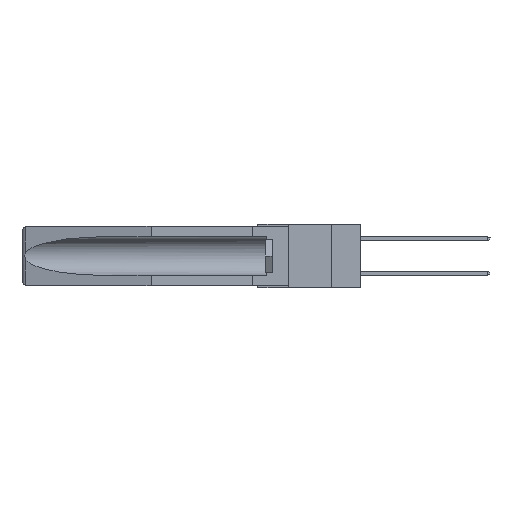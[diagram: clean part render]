
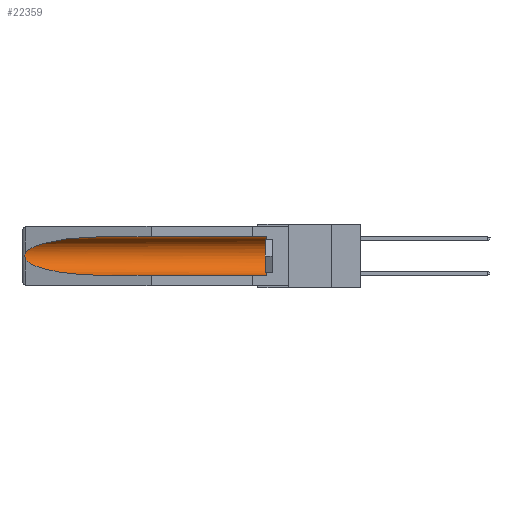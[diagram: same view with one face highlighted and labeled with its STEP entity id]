
A CAD part, left-side view. The second image highlights one B-rep face of the part: STEP entity #22359.
In plain terms, the highlighted cylindrical face has radius 2.857 mm (diameter 5.715 mm), a partial arc.
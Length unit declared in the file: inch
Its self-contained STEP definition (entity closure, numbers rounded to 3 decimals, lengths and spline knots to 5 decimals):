
#38 = ORIENTED_EDGE ( 'NONE', *, *, #10257, .T. ) ;
#1427 = AXIS2_PLACEMENT_3D ( 'NONE', #23069, #27626, #1885 ) ;
#1429 = EDGE_CURVE ( 'NONE', #13107, #6019, #18528, .T. ) ;
#1885 = DIRECTION ( 'NONE',  ( 0., 0., 1. ) ) ;
#2445 = CARTESIAN_POINT ( 'NONE',  ( 0.26537, 1.52718, -0.14972 ) ) ;
#3608 = CARTESIAN_POINT ( 'NONE',  ( 0.26537, 1.52718, -0.14972 ) ) ;
#3795 = CARTESIAN_POINT ( 'NONE',  ( 0.155, -0.30754, -0.284 ) ) ;
#4229 = VERTEX_POINT ( 'NONE', #12191 ) ;
#4608 = CARTESIAN_POINT ( 'NONE',  ( 0.2675, 1.53308, -0.16763 ) ) ;
#4626 = CARTESIAN_POINT ( 'NONE',  ( 0.155, 0.126, -0.284 ) ) ;
#5654 = LINE ( 'NONE', #3795, #27416 ) ;
#6019 = VERTEX_POINT ( 'NONE', #7406 ) ;
#6058 = CARTESIAN_POINT ( 'NONE',  ( 0.155, 1.07973, -0.284 ) ) ;
#6853 = CARTESIAN_POINT ( 'NONE',  ( 0.26597, 1.52961, -0.15275 ) ) ;
#6934 = CARTESIAN_POINT ( 'NONE',  ( 0.2673, 1.5327, -0.16383 ) ) ;
#7406 = CARTESIAN_POINT ( 'NONE',  ( 0.155, 0.126, -0.059 ) ) ;
#7929 = VERTEX_POINT ( 'NONE', #20129 ) ;
#8015 = ORIENTED_EDGE ( 'NONE', *, *, #17765, .T. ) ;
#8219 = DIRECTION ( 'NONE',  ( 0., 1., 0. ) ) ;
#8645 = CARTESIAN_POINT ( 'NONE',  ( 0.21114, 1.30732, -0.059 ) ) ;
#9231 = AXIS2_PLACEMENT_3D ( 'NONE', #27936, #21103, #23392 ) ;
#9607 = VERTEX_POINT ( 'NONE', #3608 ) ;
#10202 = EDGE_CURVE ( 'NONE', #6019, #7929, #25966, .T. ) ;
#10257 = EDGE_CURVE ( 'NONE', #9607, #19282, #23109, .T. ) ;
#10764 =( BOUNDED_CURVE ( )  B_SPLINE_CURVE ( 3, ( #17662, #8645, #13147, #21856 ),
 .UNSPECIFIED., .F., .F. ) 
 B_SPLINE_CURVE_WITH_KNOTS ( ( 4, 4 ),
 ( 4.71239, 6.08839 ),
 .UNSPECIFIED. ) 
 CURVE ( )  GEOMETRIC_REPRESENTATION_ITEM ( )  RATIONAL_B_SPLINE_CURVE ( ( 1., 0.848, 0.848, 1. ) ) 
 REPRESENTATION_ITEM ( '' )  );
#11072 = ORIENTED_EDGE ( 'NONE', *, *, #26405, .T. ) ;
#11145 = DIRECTION ( 'NONE',  ( 0., 1., 0. ) ) ;
#11305 = CARTESIAN_POINT ( 'NONE',  ( 0.2675, 1.53308, -0.17534 ) ) ;
#12184 =( BOUNDED_CURVE ( )  B_SPLINE_CURVE ( 3, ( #19154, #17029, #19353, #6058 ),
 .UNSPECIFIED., .F., .F. ) 
 B_SPLINE_CURVE_WITH_KNOTS ( ( 4, 4 ),
 ( 0.1948, 1.5708 ),
 .UNSPECIFIED. ) 
 CURVE ( )  GEOMETRIC_REPRESENTATION_ITEM ( )  RATIONAL_B_SPLINE_CURVE ( ( 1., 0.848, 0.848, 1. ) ) 
 REPRESENTATION_ITEM ( '' )  );
#12191 = CARTESIAN_POINT ( 'NONE',  ( 0.155, 1.07973, -0.284 ) ) ;
#13107 = VERTEX_POINT ( 'NONE', #4626 ) ;
#13147 = CARTESIAN_POINT ( 'NONE',  ( 0.25451, 1.48313, -0.09465 ) ) ;
#14071 = ORIENTED_EDGE ( 'NONE', *, *, #26380, .F. ) ;
#15782 = CARTESIAN_POINT ( 'NONE',  ( 0.26655, 1.53094, -0.18657 ) ) ;
#17029 = CARTESIAN_POINT ( 'NONE',  ( 0.25451, 1.48313, -0.24835 ) ) ;
#17662 = CARTESIAN_POINT ( 'NONE',  ( 0.155, 1.07973, -0.059 ) ) ;
#17765 = EDGE_CURVE ( 'NONE', #19282, #4229, #12184, .T. ) ;
#17915 = CARTESIAN_POINT ( 'NONE',  ( 0.26654, 1.53092, -0.15636 ) ) ;
#18528 = CIRCLE ( 'NONE', #9231, 0.1125 ) ;
#19154 = CARTESIAN_POINT ( 'NONE',  ( 0.26537, 1.52718, -0.19328 ) ) ;
#19282 = VERTEX_POINT ( 'NONE', #26618 ) ;
#19353 = CARTESIAN_POINT ( 'NONE',  ( 0.21114, 1.30732, -0.284 ) ) ;
#19820 = VECTOR ( 'NONE', #8219, 39.37008 ) ;
#20000 = ORIENTED_EDGE ( 'NONE', *, *, #10202, .T. ) ;
#20115 = CARTESIAN_POINT ( 'NONE',  ( 0.26537, 1.52718, -0.19328 ) ) ;
#20129 = CARTESIAN_POINT ( 'NONE',  ( 0.155, 1.07973, -0.059 ) ) ;
#21103 = DIRECTION ( 'NONE',  ( 0., -1., 0. ) ) ;
#21434 = CARTESIAN_POINT ( 'NONE',  ( 0.155, -0.30754, -0.059 ) ) ;
#21519 = FACE_OUTER_BOUND ( 'NONE', #26461, .T. ) ;
#21856 = CARTESIAN_POINT ( 'NONE',  ( 0.26537, 1.52718, -0.14972 ) ) ;
#22359 = ADVANCED_FACE ( 'NONE', ( #21519 ), #23535, .F. ) ;
#22988 = ORIENTED_EDGE ( 'NONE', *, *, #1429, .T. ) ;
#23069 = CARTESIAN_POINT ( 'NONE',  ( 0.155, -0.30754, -0.1715 ) ) ;
#23109 = B_SPLINE_CURVE_WITH_KNOTS ( 'NONE', 3,
 ( #2445, #6853, #17915, #6934, #4608, #11305, #26731, #15782, #24589, #20115 ),
 .UNSPECIFIED., .F., .F.,
 ( 4, 2, 2, 2, 4 ),
 ( 0., 0.00029, 0.00058, 0.00087, 0.00117 ),
 .UNSPECIFIED. ) ;
#23392 = DIRECTION ( 'NONE',  ( 0., 0., 1. ) ) ;
#23535 = CYLINDRICAL_SURFACE ( 'NONE', #1427, 0.1125 ) ;
#24589 = CARTESIAN_POINT ( 'NONE',  ( 0.26597, 1.5296, -0.19026 ) ) ;
#25966 = LINE ( 'NONE', #21434, #19820 ) ;
#26380 = EDGE_CURVE ( 'NONE', #13107, #4229, #5654, .T. ) ;
#26405 = EDGE_CURVE ( 'NONE', #7929, #9607, #10764, .T. ) ;
#26461 = EDGE_LOOP ( 'NONE', ( #11072, #38, #8015, #14071, #22988, #20000 ) ) ;
#26618 = CARTESIAN_POINT ( 'NONE',  ( 0.26537, 1.52718, -0.19328 ) ) ;
#26731 = CARTESIAN_POINT ( 'NONE',  ( 0.2673, 1.53269, -0.17917 ) ) ;
#27416 = VECTOR ( 'NONE', #11145, 39.37008 ) ;
#27626 = DIRECTION ( 'NONE',  ( 0., 1., 0. ) ) ;
#27936 = CARTESIAN_POINT ( 'NONE',  ( 0.155, 0.126, -0.1715 ) ) ;
